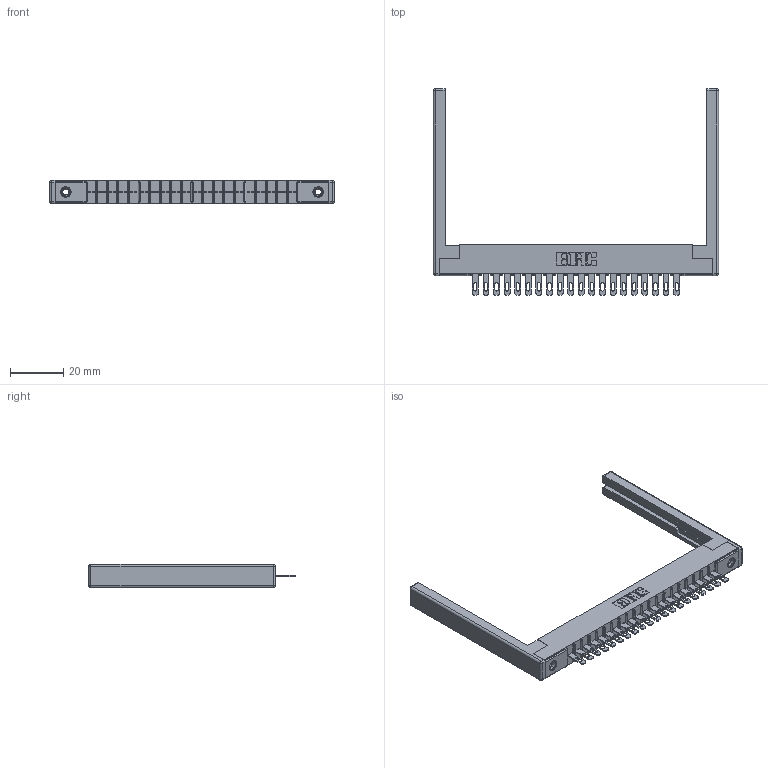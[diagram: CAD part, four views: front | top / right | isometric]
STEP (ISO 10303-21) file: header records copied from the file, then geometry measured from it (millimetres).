
FILE_DESCRIPTION (( 'STEP AP203' ), '1' );
FILE_NAME ('356-020-400-168.STEP', '2020-09-23T14:21:34', ( '' ), ( '' ), 'SwSTEP 2.0', 'SolidWorks 2020', '' );
FILE_SCHEMA (( 'CONFIG_CONTROL_DESIGN' ));
Length unit declared in the file: inch
Products named in the file (5): 345-250-001_345-250-001-102; 306-290-001_100; 306 Part_.156 Dia; 307-220-068; 356-020-400-168
Assembly tree (25 placements, depth 2):
  356-020-400-168
    306 Part_.156 Dia
    306-290-001_100  x20
    345-250-001_345-250-001-102  x2
    307-220-068  x2
Bounding box: 106.68 x 77.17 x 8.71 mm (x, y, z)
Volume: 11895.9 mm3; surface area: 15240.6 mm2
Topology: 25 solids, 25 shells, 1790 faces, 5006 edges, 3208 vertices
Faces by surface type: plane 1156, cylinder 530, sphere 88, cone 12, torus 4
Entity records: 24424 total; most frequent: CARTESIAN_POINT 4064, DIRECTION 4023, ORIENTED_EDGE 4018, EDGE_CURVE 2009, VECTOR 1553, LINE 1553, VERTEX_POINT 1276, AXIS2_PLACEMENT_3D 1235
